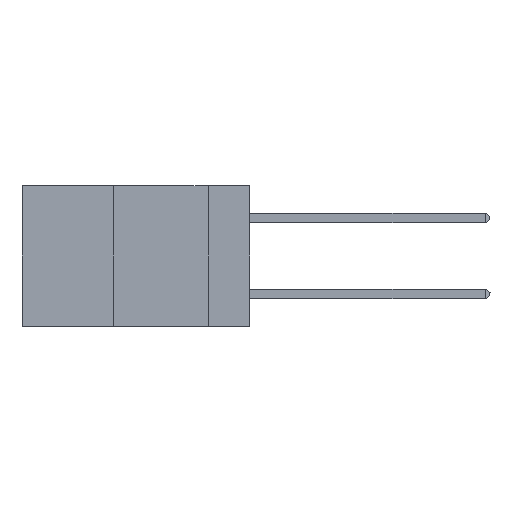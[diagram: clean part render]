
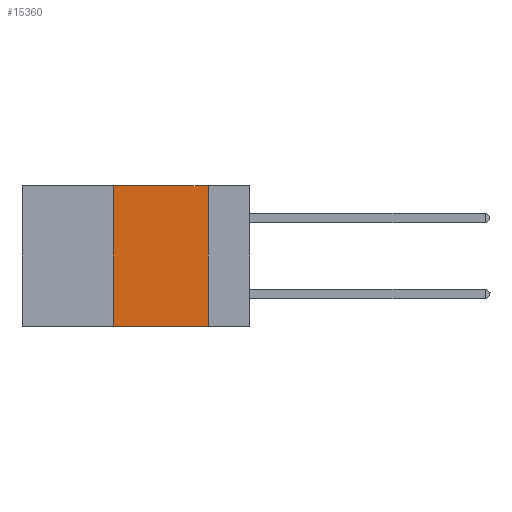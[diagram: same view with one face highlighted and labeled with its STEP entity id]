
A CAD part, left-side view. The second image highlights one B-rep face of the part: STEP entity #15360.
In plain terms, the highlighted planar face has unit normal (-1, 0, 0).
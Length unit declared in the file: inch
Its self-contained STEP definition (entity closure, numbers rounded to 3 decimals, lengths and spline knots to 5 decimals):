
#1645 = VECTOR ( 'NONE', #11325, 39.37008 ) ;
#3259 = EDGE_LOOP ( 'NONE', ( #30862, #34786, #10456, #26200 ) ) ;
#3539 = CARTESIAN_POINT ( 'NONE',  ( 0., 0.11, 0. ) ) ;
#4267 = DIRECTION ( 'NONE',  ( 0., 0., -1. ) ) ;
#4398 = DIRECTION ( 'NONE',  ( 0., 0., -1. ) ) ;
#5592 = VECTOR ( 'NONE', #25451, 39.37008 ) ;
#6315 = VERTEX_POINT ( 'NONE', #17066 ) ;
#7876 = EDGE_CURVE ( 'NONE', #36160, #35725, #15525, .T. ) ;
#10456 = ORIENTED_EDGE ( 'NONE', *, *, #11746, .F. ) ;
#10639 = VECTOR ( 'NONE', #19055, 39.37008 ) ;
#10937 = CARTESIAN_POINT ( 'NONE',  ( 0., 0.36, -0.37 ) ) ;
#11325 = DIRECTION ( 'NONE',  ( 0., -1., 0. ) ) ;
#11341 = LINE ( 'NONE', #3539, #37026 ) ;
#11746 = EDGE_CURVE ( 'NONE', #42392, #36160, #33679, .T. ) ;
#11819 = CARTESIAN_POINT ( 'NONE',  ( 0., 0.6, 0. ) ) ;
#12501 = CARTESIAN_POINT ( 'NONE',  ( 0., 0.36, 0. ) ) ;
#15360 = ADVANCED_FACE ( 'NONE', ( #32334 ), #27289, .F. ) ;
#15525 = LINE ( 'NONE', #11819, #5592 ) ;
#16809 = CARTESIAN_POINT ( 'NONE',  ( 0., 0.6, 0. ) ) ;
#17066 = CARTESIAN_POINT ( 'NONE',  ( 0., 0.11, -0.37 ) ) ;
#19055 = DIRECTION ( 'NONE',  ( 0., 0., 1. ) ) ;
#23090 = CARTESIAN_POINT ( 'NONE',  ( 0., 0.11, 0. ) ) ;
#25451 = DIRECTION ( 'NONE',  ( 0., -1., 0. ) ) ;
#25981 = CARTESIAN_POINT ( 'NONE',  ( 0., 0.36, 0. ) ) ;
#26200 = ORIENTED_EDGE ( 'NONE', *, *, #27099, .T. ) ;
#27099 = EDGE_CURVE ( 'NONE', #42392, #6315, #28923, .T. ) ;
#27289 = PLANE ( 'NONE',  #29524 ) ;
#28923 = LINE ( 'NONE', #37557, #1645 ) ;
#29524 = AXIS2_PLACEMENT_3D ( 'NONE', #16809, #40294, #4398 ) ;
#30862 = ORIENTED_EDGE ( 'NONE', *, *, #36539, .F. ) ;
#32334 = FACE_OUTER_BOUND ( 'NONE', #3259, .T. ) ;
#33679 = LINE ( 'NONE', #25981, #10639 ) ;
#34786 = ORIENTED_EDGE ( 'NONE', *, *, #7876, .F. ) ;
#35725 = VERTEX_POINT ( 'NONE', #23090 ) ;
#36160 = VERTEX_POINT ( 'NONE', #12501 ) ;
#36539 = EDGE_CURVE ( 'NONE', #35725, #6315, #11341, .T. ) ;
#37026 = VECTOR ( 'NONE', #4267, 39.37008 ) ;
#37557 = CARTESIAN_POINT ( 'NONE',  ( 0., 0.6, -0.37 ) ) ;
#40294 = DIRECTION ( 'NONE',  ( 1., 0., 0. ) ) ;
#42392 = VERTEX_POINT ( 'NONE', #10937 ) ;
